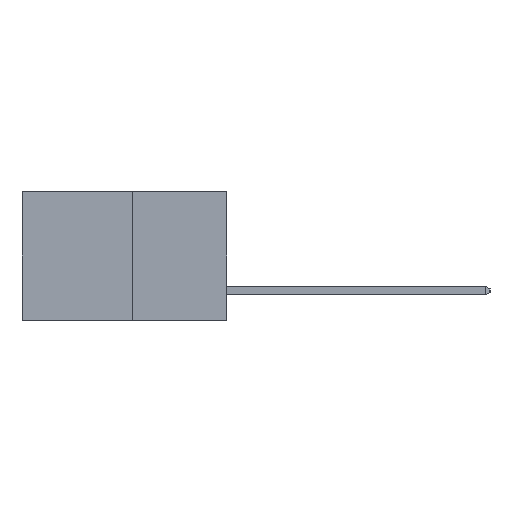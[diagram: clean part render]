
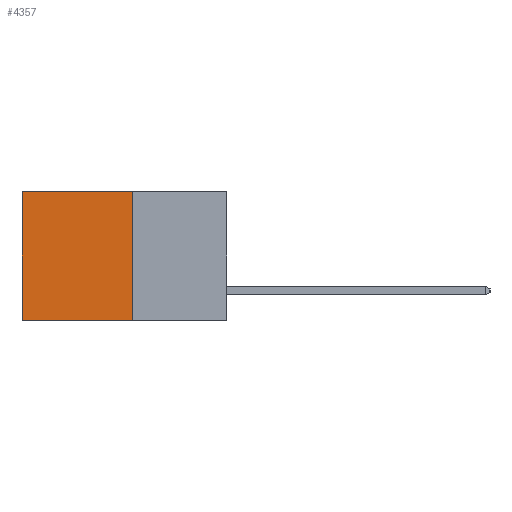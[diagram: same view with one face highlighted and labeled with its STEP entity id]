
A CAD part, left-side view. The second image highlights one B-rep face of the part: STEP entity #4357.
In plain terms, the highlighted planar face has unit normal (-1, 0, 0).
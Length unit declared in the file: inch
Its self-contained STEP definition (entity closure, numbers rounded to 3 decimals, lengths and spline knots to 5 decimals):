
#740 = VERTEX_POINT ( 'NONE', #9024 ) ;
#787 = ORIENTED_EDGE ( 'NONE', *, *, #4823, .F. ) ;
#1332 = ORIENTED_EDGE ( 'NONE', *, *, #8459, .T. ) ;
#1930 = CARTESIAN_POINT ( 'NONE',  ( 0.277, 0.27, -0.37 ) ) ;
#2149 = DIRECTION ( 'NONE',  ( 0., 1., 0. ) ) ;
#2164 = DIRECTION ( 'NONE',  ( 0., 0., -1. ) ) ;
#2337 = EDGE_LOOP ( 'NONE', ( #8874, #787, #10371, #1332 ) ) ;
#2664 = LINE ( 'NONE', #7989, #7080 ) ;
#3076 = VERTEX_POINT ( 'NONE', #9020 ) ;
#3300 = DIRECTION ( 'NONE',  ( 0., 0., -1. ) ) ;
#3460 = CARTESIAN_POINT ( 'NONE',  ( 0.277, 0.27, 0. ) ) ;
#4139 = CARTESIAN_POINT ( 'NONE',  ( 0.277, 0.59, -0.37 ) ) ;
#4152 = EDGE_CURVE ( 'NONE', #4626, #5585, #7544, .T. ) ;
#4357 = ADVANCED_FACE ( 'NONE', ( #9489 ), #7630, .F. ) ;
#4626 = VERTEX_POINT ( 'NONE', #3460 ) ;
#4691 = DIRECTION ( 'NONE',  ( 0., 1., 0. ) ) ;
#4823 = EDGE_CURVE ( 'NONE', #5585, #740, #7792, .T. ) ;
#4901 = CARTESIAN_POINT ( 'NONE',  ( 0.277, 0.27, -0.37 ) ) ;
#4981 = CARTESIAN_POINT ( 'NONE',  ( 0.277, 0.27, -0.37 ) ) ;
#5251 = DIRECTION ( 'NONE',  ( 0., 0., -1. ) ) ;
#5585 = VERTEX_POINT ( 'NONE', #7495 ) ;
#6329 = LINE ( 'NONE', #4139, #10298 ) ;
#7080 = VECTOR ( 'NONE', #2149, 39.37008 ) ;
#7495 = CARTESIAN_POINT ( 'NONE',  ( 0.277, 0.27, -0.37 ) ) ;
#7544 = LINE ( 'NONE', #1930, #9371 ) ;
#7630 = PLANE ( 'NONE',  #8802 ) ;
#7719 = DIRECTION ( 'NONE',  ( 1., 0., 0. ) ) ;
#7792 = LINE ( 'NONE', #4901, #9870 ) ;
#7989 = CARTESIAN_POINT ( 'NONE',  ( 0.277, 0.27, 0. ) ) ;
#8131 = EDGE_CURVE ( 'NONE', #3076, #740, #6329, .T. ) ;
#8459 = EDGE_CURVE ( 'NONE', #4626, #3076, #2664, .T. ) ;
#8802 = AXIS2_PLACEMENT_3D ( 'NONE', #4981, #7719, #5251 ) ;
#8874 = ORIENTED_EDGE ( 'NONE', *, *, #8131, .T. ) ;
#9020 = CARTESIAN_POINT ( 'NONE',  ( 0.277, 0.59, 0. ) ) ;
#9024 = CARTESIAN_POINT ( 'NONE',  ( 0.277, 0.59, -0.37 ) ) ;
#9371 = VECTOR ( 'NONE', #2164, 39.37008 ) ;
#9489 = FACE_OUTER_BOUND ( 'NONE', #2337, .T. ) ;
#9870 = VECTOR ( 'NONE', #4691, 39.37008 ) ;
#10298 = VECTOR ( 'NONE', #3300, 39.37008 ) ;
#10371 = ORIENTED_EDGE ( 'NONE', *, *, #4152, .F. ) ;
